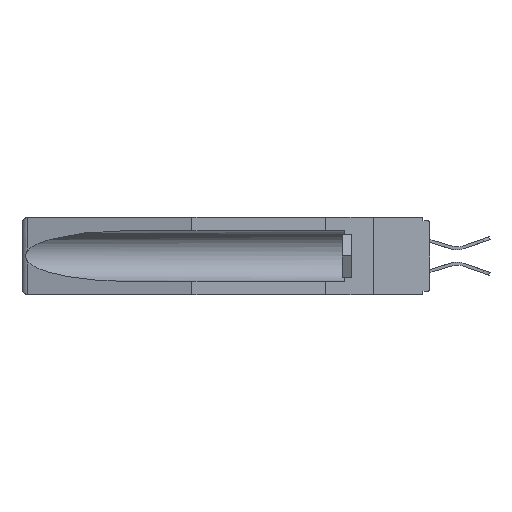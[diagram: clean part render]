
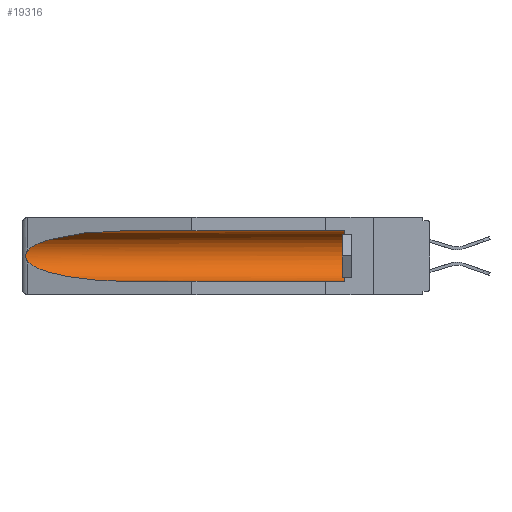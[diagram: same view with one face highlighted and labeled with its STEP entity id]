
A CAD part, left-side view. The second image highlights one B-rep face of the part: STEP entity #19316.
In plain terms, the highlighted cylindrical face has radius 2.857 mm (diameter 5.715 mm), a partial arc.
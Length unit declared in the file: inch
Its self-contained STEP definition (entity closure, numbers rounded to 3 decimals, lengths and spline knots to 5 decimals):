
#247 = EDGE_CURVE ( 'NONE', #13153, #15508, #5027, .T. ) ;
#380 = CARTESIAN_POINT ( 'NONE',  ( 0.155, 0.126, -0.284 ) ) ;
#1078 = EDGE_CURVE ( 'NONE', #17878, #13153, #13514, .T. ) ;
#1539 = ORIENTED_EDGE ( 'NONE', *, *, #12471, .F. ) ;
#1622 = B_SPLINE_CURVE_WITH_KNOTS ( 'NONE', 3,
 ( #9192, #10193, #18712, #5504, #5986, #11827, #3849, #10321, #12305, #19913 ),
 .UNSPECIFIED., .F., .F.,
 ( 4, 2, 2, 2, 4 ),
 ( 0., 0.00029, 0.00058, 0.00087, 0.00117 ),
 .UNSPECIFIED. ) ;
#1924 = CARTESIAN_POINT ( 'NONE',  ( 0.155, -0.30754, -0.1715 ) ) ;
#2367 = CARTESIAN_POINT ( 'NONE',  ( 0.155, -0.30754, -0.059 ) ) ;
#2565 = CARTESIAN_POINT ( 'NONE',  ( 0.155, -0.30754, -0.284 ) ) ;
#2808 = VERTEX_POINT ( 'NONE', #10451 ) ;
#2811 = VERTEX_POINT ( 'NONE', #14201 ) ;
#3128 = EDGE_CURVE ( 'NONE', #2808, #2811, #1622, .T. ) ;
#3132 = LINE ( 'NONE', #2565, #19922 ) ;
#3155 = DIRECTION ( 'NONE',  ( 0., 0., 1. ) ) ;
#3675 = CARTESIAN_POINT ( 'NONE',  ( 0.155, 0.126, -0.059 ) ) ;
#3849 = CARTESIAN_POINT ( 'NONE',  ( 0.2673, 1.53269, -0.17917 ) ) ;
#3870 = DIRECTION ( 'NONE',  ( 0., 1., 0. ) ) ;
#4210 = FACE_OUTER_BOUND ( 'NONE', #5384, .T. ) ;
#4845 = CARTESIAN_POINT ( 'NONE',  ( 0.26537, 1.52718, -0.14972 ) ) ;
#5027 = LINE ( 'NONE', #2367, #16051 ) ;
#5384 = EDGE_LOOP ( 'NONE', ( #11235, #12322, #16256, #1539, #11171, #10735 ) ) ;
#5504 = CARTESIAN_POINT ( 'NONE',  ( 0.2673, 1.5327, -0.16383 ) ) ;
#5912 = CARTESIAN_POINT ( 'NONE',  ( 0.25451, 1.48313, -0.09465 ) ) ;
#5986 = CARTESIAN_POINT ( 'NONE',  ( 0.2675, 1.53308, -0.16763 ) ) ;
#9192 = CARTESIAN_POINT ( 'NONE',  ( 0.26537, 1.52718, -0.14972 ) ) ;
#9514 = DIRECTION ( 'NONE',  ( 0., -1., 0. ) ) ;
#9592 = CARTESIAN_POINT ( 'NONE',  ( 0.26537, 1.52718, -0.19328 ) ) ;
#10193 = CARTESIAN_POINT ( 'NONE',  ( 0.26597, 1.52961, -0.15275 ) ) ;
#10321 = CARTESIAN_POINT ( 'NONE',  ( 0.26655, 1.53094, -0.18657 ) ) ;
#10451 = CARTESIAN_POINT ( 'NONE',  ( 0.26537, 1.52718, -0.14972 ) ) ;
#10735 = ORIENTED_EDGE ( 'NONE', *, *, #247, .T. ) ;
#11134 = CARTESIAN_POINT ( 'NONE',  ( 0.155, 0.126, -0.1715 ) ) ;
#11171 = ORIENTED_EDGE ( 'NONE', *, *, #1078, .T. ) ;
#11235 = ORIENTED_EDGE ( 'NONE', *, *, #13112, .T. ) ;
#11447 = EDGE_CURVE ( 'NONE', #2811, #14379, #18651, .T. ) ;
#11827 = CARTESIAN_POINT ( 'NONE',  ( 0.2675, 1.53308, -0.17534 ) ) ;
#12215 = CYLINDRICAL_SURFACE ( 'NONE', #13558, 0.1125 ) ;
#12305 = CARTESIAN_POINT ( 'NONE',  ( 0.26597, 1.5296, -0.19026 ) ) ;
#12322 = ORIENTED_EDGE ( 'NONE', *, *, #3128, .T. ) ;
#12471 = EDGE_CURVE ( 'NONE', #17878, #14379, #3132, .T. ) ;
#13112 = EDGE_CURVE ( 'NONE', #15508, #2808, #14995, .T. ) ;
#13153 = VERTEX_POINT ( 'NONE', #3675 ) ;
#13514 = CIRCLE ( 'NONE', #13775, 0.1125 ) ;
#13558 = AXIS2_PLACEMENT_3D ( 'NONE', #1924, #3870, #18456 ) ;
#13775 = AXIS2_PLACEMENT_3D ( 'NONE', #11134, #9514, #3155 ) ;
#14201 = CARTESIAN_POINT ( 'NONE',  ( 0.26537, 1.52718, -0.19328 ) ) ;
#14379 = VERTEX_POINT ( 'NONE', #16112 ) ;
#14995 =( BOUNDED_CURVE ( )  B_SPLINE_CURVE ( 3, ( #17246, #18911, #5912, #4845 ),
 .UNSPECIFIED., .F., .F. ) 
 B_SPLINE_CURVE_WITH_KNOTS ( ( 4, 4 ),
 ( 4.71239, 6.08839 ),
 .UNSPECIFIED. ) 
 CURVE ( )  GEOMETRIC_REPRESENTATION_ITEM ( )  RATIONAL_B_SPLINE_CURVE ( ( 1., 0.848, 0.848, 1. ) ) 
 REPRESENTATION_ITEM ( '' )  );
#15209 = DIRECTION ( 'NONE',  ( 0., 1., 0. ) ) ;
#15508 = VERTEX_POINT ( 'NONE', #17649 ) ;
#16051 = VECTOR ( 'NONE', #15209, 39.37008 ) ;
#16112 = CARTESIAN_POINT ( 'NONE',  ( 0.155, 1.07973, -0.284 ) ) ;
#16256 = ORIENTED_EDGE ( 'NONE', *, *, #11447, .T. ) ;
#17061 = DIRECTION ( 'NONE',  ( 0., 1., 0. ) ) ;
#17246 = CARTESIAN_POINT ( 'NONE',  ( 0.155, 1.07973, -0.059 ) ) ;
#17498 = CARTESIAN_POINT ( 'NONE',  ( 0.25451, 1.48313, -0.24835 ) ) ;
#17649 = CARTESIAN_POINT ( 'NONE',  ( 0.155, 1.07973, -0.059 ) ) ;
#17878 = VERTEX_POINT ( 'NONE', #380 ) ;
#18456 = DIRECTION ( 'NONE',  ( 0., 0., 1. ) ) ;
#18651 =( BOUNDED_CURVE ( )  B_SPLINE_CURVE ( 3, ( #9592, #17498, #19102, #20701 ),
 .UNSPECIFIED., .F., .F. ) 
 B_SPLINE_CURVE_WITH_KNOTS ( ( 4, 4 ),
 ( 0.1948, 1.5708 ),
 .UNSPECIFIED. ) 
 CURVE ( )  GEOMETRIC_REPRESENTATION_ITEM ( )  RATIONAL_B_SPLINE_CURVE ( ( 1., 0.848, 0.848, 1. ) ) 
 REPRESENTATION_ITEM ( '' )  );
#18712 = CARTESIAN_POINT ( 'NONE',  ( 0.26654, 1.53092, -0.15636 ) ) ;
#18911 = CARTESIAN_POINT ( 'NONE',  ( 0.21114, 1.30732, -0.059 ) ) ;
#19102 = CARTESIAN_POINT ( 'NONE',  ( 0.21114, 1.30732, -0.284 ) ) ;
#19316 = ADVANCED_FACE ( 'NONE', ( #4210 ), #12215, .F. ) ;
#19913 = CARTESIAN_POINT ( 'NONE',  ( 0.26537, 1.52718, -0.19328 ) ) ;
#19922 = VECTOR ( 'NONE', #17061, 39.37008 ) ;
#20701 = CARTESIAN_POINT ( 'NONE',  ( 0.155, 1.07973, -0.284 ) ) ;
